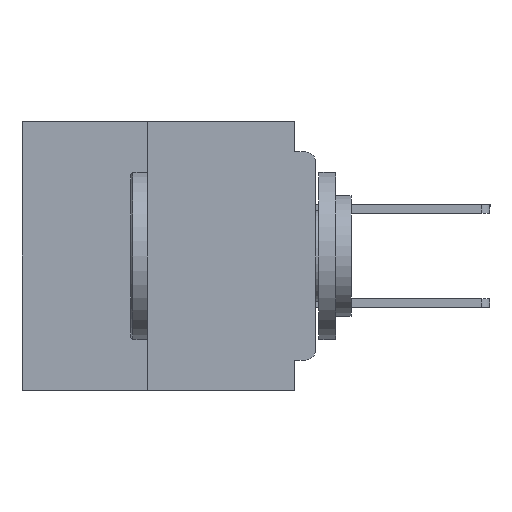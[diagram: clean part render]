
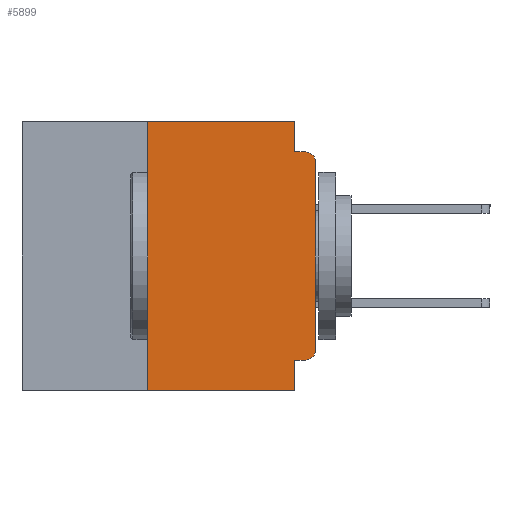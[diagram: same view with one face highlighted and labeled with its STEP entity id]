
A CAD part, left-side view. The second image highlights one B-rep face of the part: STEP entity #5899.
In plain terms, the highlighted planar face has unit normal (-1, 0, 0).
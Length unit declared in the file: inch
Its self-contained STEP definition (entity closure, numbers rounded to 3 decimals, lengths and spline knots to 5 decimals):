
#84 = VECTOR ( 'NONE', #17444, 39.37008 ) ;
#1583 = VECTOR ( 'NONE', #46526, 39.37008 ) ;
#1666 = ORIENTED_EDGE ( 'NONE', *, *, #13791, .T. ) ;
#1888 = VERTEX_POINT ( 'NONE', #20959 ) ;
#2217 = VERTEX_POINT ( 'NONE', #25836 ) ;
#2316 = CARTESIAN_POINT ( 'NONE',  ( 0., 0.031, 0. ) ) ;
#3675 = CARTESIAN_POINT ( 'NONE',  ( 0., 0., 0. ) ) ;
#4099 = CARTESIAN_POINT ( 'NONE',  ( 0., 0.25, -0.4 ) ) ;
#4783 = LINE ( 'NONE', #45688, #39410 ) ;
#5688 = ORIENTED_EDGE ( 'NONE', *, *, #49952, .T. ) ;
#5899 = ADVANCED_FACE ( 'NONE', ( #20438 ), #35235, .F. ) ;
#6057 = DIRECTION ( 'NONE',  ( -1., 0., 0. ) ) ;
#7202 = VERTEX_POINT ( 'NONE', #4099 ) ;
#8243 = CARTESIAN_POINT ( 'NONE',  ( 0., 0.437, 0. ) ) ;
#9292 = VECTOR ( 'NONE', #41605, 39.37008 ) ;
#9596 = EDGE_CURVE ( 'NONE', #22303, #20099, #23773, .T. ) ;
#10058 = CARTESIAN_POINT ( 'NONE',  ( 0., 0.031, 0. ) ) ;
#10839 = ORIENTED_EDGE ( 'NONE', *, *, #57524, .F. ) ;
#12180 = LINE ( 'NONE', #3675, #84 ) ;
#12845 = DIRECTION ( 'NONE',  ( 1., 0., 0. ) ) ;
#12937 = CARTESIAN_POINT ( 'NONE',  ( 0., 0., -0.355 ) ) ;
#13370 = CARTESIAN_POINT ( 'NONE',  ( 0., 0.031, -0.355 ) ) ;
#13377 = CIRCLE ( 'NONE', #18390, 0.015 ) ;
#13791 = EDGE_CURVE ( 'NONE', #22303, #23806, #13377, .T. ) ;
#14369 = EDGE_CURVE ( 'NONE', #7202, #2217, #25967, .T. ) ;
#15494 = ORIENTED_EDGE ( 'NONE', *, *, #9596, .F. ) ;
#15875 = EDGE_CURVE ( 'NONE', #37064, #32774, #4783, .T. ) ;
#16266 = VERTEX_POINT ( 'NONE', #57283 ) ;
#16682 = ORIENTED_EDGE ( 'NONE', *, *, #41522, .F. ) ;
#17444 = DIRECTION ( 'NONE',  ( 0., 0., 1. ) ) ;
#17479 = DIRECTION ( 'NONE',  ( 0., 1., 0. ) ) ;
#18057 = CARTESIAN_POINT ( 'NONE',  ( 0., 0.031, -0.4 ) ) ;
#18390 = AXIS2_PLACEMENT_3D ( 'NONE', #46566, #19708, #51070 ) ;
#18545 = LINE ( 'NONE', #10058, #9292 ) ;
#19539 = EDGE_CURVE ( 'NONE', #23806, #20638, #12180, .T. ) ;
#19708 = DIRECTION ( 'NONE',  ( -1., 0., 0. ) ) ;
#19847 = CARTESIAN_POINT ( 'NONE',  ( 0., 0.25, -0.4 ) ) ;
#20099 = VERTEX_POINT ( 'NONE', #13370 ) ;
#20438 = FACE_OUTER_BOUND ( 'NONE', #40644, .T. ) ;
#20638 = VERTEX_POINT ( 'NONE', #48475 ) ;
#20959 = CARTESIAN_POINT ( 'NONE',  ( 0., 0.031, -0.045 ) ) ;
#21834 = LINE ( 'NONE', #35895, #32332 ) ;
#22042 = ORIENTED_EDGE ( 'NONE', *, *, #15875, .F. ) ;
#22303 = VERTEX_POINT ( 'NONE', #25137 ) ;
#23773 = LINE ( 'NONE', #12937, #47652 ) ;
#23806 = VERTEX_POINT ( 'NONE', #32154 ) ;
#25137 = CARTESIAN_POINT ( 'NONE',  ( 0., 0.015, -0.355 ) ) ;
#25205 = AXIS2_PLACEMENT_3D ( 'NONE', #33071, #6057, #37610 ) ;
#25374 = DIRECTION ( 'NONE',  ( 0., -1., 0. ) ) ;
#25836 = CARTESIAN_POINT ( 'NONE',  ( 0., 0.031, -0.4 ) ) ;
#25967 = LINE ( 'NONE', #29881, #27382 ) ;
#26384 = LINE ( 'NONE', #18057, #36933 ) ;
#27382 = VECTOR ( 'NONE', #25374, 39.37008 ) ;
#29881 = CARTESIAN_POINT ( 'NONE',  ( 0., 0.437, -0.4 ) ) ;
#32154 = CARTESIAN_POINT ( 'NONE',  ( 0., 0., -0.34 ) ) ;
#32332 = VECTOR ( 'NONE', #40458, 39.37008 ) ;
#32774 = VERTEX_POINT ( 'NONE', #2316 ) ;
#33071 = CARTESIAN_POINT ( 'NONE',  ( 0., 0.015, -0.06 ) ) ;
#35235 = PLANE ( 'NONE',  #50467 ) ;
#35431 = EDGE_CURVE ( 'NONE', #7202, #37064, #39110, .T. ) ;
#35895 = CARTESIAN_POINT ( 'NONE',  ( 0., 0., -0.045 ) ) ;
#36933 = VECTOR ( 'NONE', #58370, 39.37008 ) ;
#37064 = VERTEX_POINT ( 'NONE', #45190 ) ;
#37610 = DIRECTION ( 'NONE',  ( 0., 0., -1. ) ) ;
#39110 = LINE ( 'NONE', #19847, #1583 ) ;
#39410 = VECTOR ( 'NONE', #41193, 39.37008 ) ;
#40298 = ORIENTED_EDGE ( 'NONE', *, *, #35431, .F. ) ;
#40458 = DIRECTION ( 'NONE',  ( 0., -1., 0. ) ) ;
#40644 = EDGE_LOOP ( 'NONE', ( #44491, #5688, #45777, #16682, #22042, #40298, #48882, #10839, #15494, #1666 ) ) ;
#41193 = DIRECTION ( 'NONE',  ( 0., -1., 0. ) ) ;
#41522 = EDGE_CURVE ( 'NONE', #32774, #1888, #18545, .T. ) ;
#41605 = DIRECTION ( 'NONE',  ( 0., 0., -1. ) ) ;
#44305 = DIRECTION ( 'NONE',  ( 0., 0., -1. ) ) ;
#44491 = ORIENTED_EDGE ( 'NONE', *, *, #19539, .T. ) ;
#45190 = CARTESIAN_POINT ( 'NONE',  ( 0., 0.25, 0. ) ) ;
#45688 = CARTESIAN_POINT ( 'NONE',  ( 0., 0.437, 0. ) ) ;
#45777 = ORIENTED_EDGE ( 'NONE', *, *, #54798, .F. ) ;
#46526 = DIRECTION ( 'NONE',  ( 0., 0., 1. ) ) ;
#46566 = CARTESIAN_POINT ( 'NONE',  ( 0., 0.015, -0.34 ) ) ;
#47652 = VECTOR ( 'NONE', #17479, 39.37008 ) ;
#48475 = CARTESIAN_POINT ( 'NONE',  ( 0., 0., -0.06 ) ) ;
#48882 = ORIENTED_EDGE ( 'NONE', *, *, #14369, .T. ) ;
#49952 = EDGE_CURVE ( 'NONE', #20638, #16266, #51665, .T. ) ;
#50467 = AXIS2_PLACEMENT_3D ( 'NONE', #8243, #12845, #44305 ) ;
#51070 = DIRECTION ( 'NONE',  ( 0., 0., -1. ) ) ;
#51665 = CIRCLE ( 'NONE', #25205, 0.015 ) ;
#54798 = EDGE_CURVE ( 'NONE', #1888, #16266, #21834, .T. ) ;
#57283 = CARTESIAN_POINT ( 'NONE',  ( 0., 0.015, -0.045 ) ) ;
#57524 = EDGE_CURVE ( 'NONE', #20099, #2217, #26384, .T. ) ;
#58370 = DIRECTION ( 'NONE',  ( 0., 0., -1. ) ) ;
